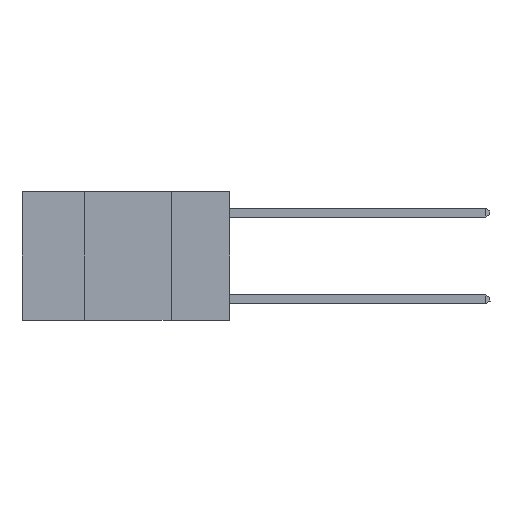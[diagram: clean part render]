
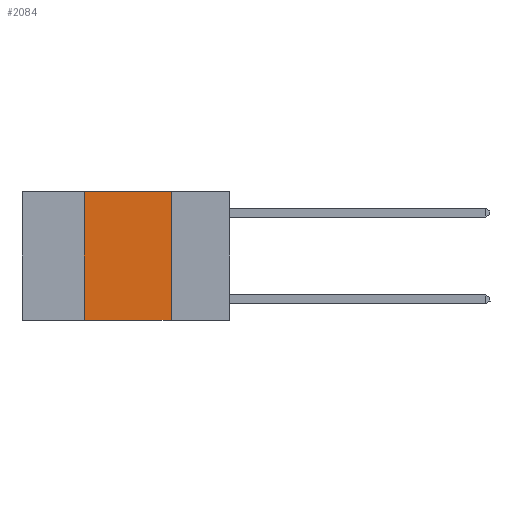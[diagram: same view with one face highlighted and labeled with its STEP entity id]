
A CAD part, left-side view. The second image highlights one B-rep face of the part: STEP entity #2084.
In plain terms, the highlighted planar face has unit normal (-1, 0, 0).
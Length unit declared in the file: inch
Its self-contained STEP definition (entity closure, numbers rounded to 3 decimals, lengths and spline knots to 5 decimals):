
#1271 = EDGE_CURVE ( 'NONE', #20536, #14595, #14914, .T. ) ;
#1341 = DIRECTION ( 'NONE',  ( 0., 0., -1. ) ) ;
#1417 = CARTESIAN_POINT ( 'NONE',  ( 0., 0.42, 0. ) ) ;
#2084 = ADVANCED_FACE ( 'NONE', ( #22231 ), #8075, .F. ) ;
#2366 = DIRECTION ( 'NONE',  ( 0., 0., -1. ) ) ;
#3370 = ORIENTED_EDGE ( 'NONE', *, *, #20392, .F. ) ;
#3470 = AXIS2_PLACEMENT_3D ( 'NONE', #18250, #14467, #2366 ) ;
#5164 = ORIENTED_EDGE ( 'NONE', *, *, #19191, .T. ) ;
#5372 = VECTOR ( 'NONE', #16043, 39.37008 ) ;
#5464 = CARTESIAN_POINT ( 'NONE',  ( 0., 0.6, -0.37 ) ) ;
#6503 = VERTEX_POINT ( 'NONE', #14824 ) ;
#8075 = PLANE ( 'NONE',  #3470 ) ;
#8445 = VECTOR ( 'NONE', #18193, 39.37008 ) ;
#8658 = VERTEX_POINT ( 'NONE', #11507 ) ;
#9481 = CARTESIAN_POINT ( 'NONE',  ( 0., 0.6, 0. ) ) ;
#9960 = LINE ( 'NONE', #5464, #23856 ) ;
#11507 = CARTESIAN_POINT ( 'NONE',  ( 0., 0.42, 0. ) ) ;
#13184 = CARTESIAN_POINT ( 'NONE',  ( 0., 0.17, 0. ) ) ;
#13678 = CARTESIAN_POINT ( 'NONE',  ( 0., 0.17, 0. ) ) ;
#14347 = VECTOR ( 'NONE', #1341, 39.37008 ) ;
#14467 = DIRECTION ( 'NONE',  ( 1., 0., 0. ) ) ;
#14522 = EDGE_CURVE ( 'NONE', #8658, #20536, #20637, .T. ) ;
#14595 = VERTEX_POINT ( 'NONE', #22727 ) ;
#14824 = CARTESIAN_POINT ( 'NONE',  ( 0., 0.42, -0.37 ) ) ;
#14843 = DIRECTION ( 'NONE',  ( 0., -1., 0. ) ) ;
#14914 = LINE ( 'NONE', #13678, #14347 ) ;
#16043 = DIRECTION ( 'NONE',  ( 0., -1., 0. ) ) ;
#18193 = DIRECTION ( 'NONE',  ( 0., 0., 1. ) ) ;
#18250 = CARTESIAN_POINT ( 'NONE',  ( 0., 0.6, 0. ) ) ;
#19103 = EDGE_LOOP ( 'NONE', ( #20709, #21265, #3370, #5164 ) ) ;
#19191 = EDGE_CURVE ( 'NONE', #6503, #14595, #9960, .T. ) ;
#20392 = EDGE_CURVE ( 'NONE', #6503, #8658, #22943, .T. ) ;
#20536 = VERTEX_POINT ( 'NONE', #13184 ) ;
#20637 = LINE ( 'NONE', #9481, #5372 ) ;
#20709 = ORIENTED_EDGE ( 'NONE', *, *, #1271, .F. ) ;
#21265 = ORIENTED_EDGE ( 'NONE', *, *, #14522, .F. ) ;
#22231 = FACE_OUTER_BOUND ( 'NONE', #19103, .T. ) ;
#22727 = CARTESIAN_POINT ( 'NONE',  ( 0., 0.17, -0.37 ) ) ;
#22943 = LINE ( 'NONE', #1417, #8445 ) ;
#23856 = VECTOR ( 'NONE', #14843, 39.37008 ) ;
